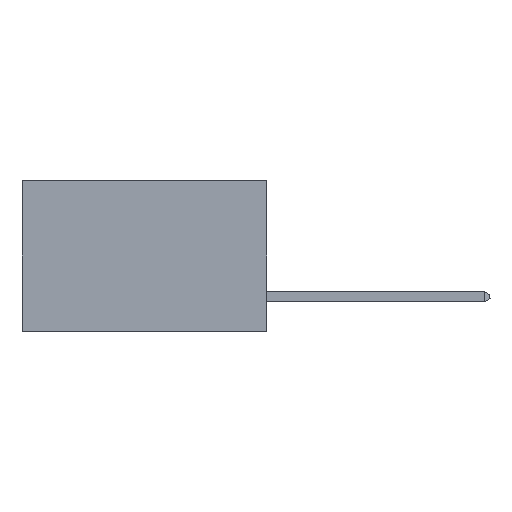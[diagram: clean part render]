
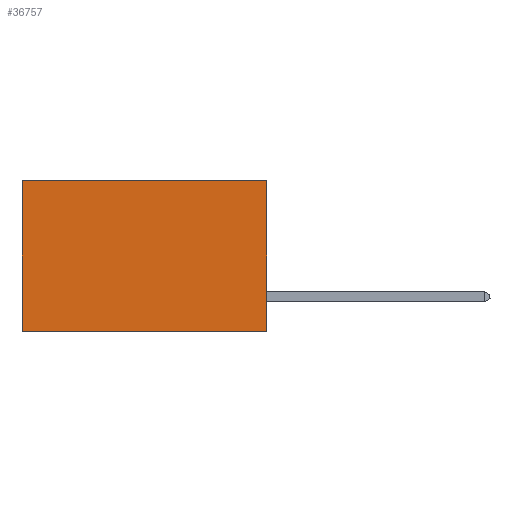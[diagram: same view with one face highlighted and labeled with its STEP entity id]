
A CAD part, left-side view. The second image highlights one B-rep face of the part: STEP entity #36757.
In plain terms, the highlighted planar face has unit normal (-1, 0, 0).
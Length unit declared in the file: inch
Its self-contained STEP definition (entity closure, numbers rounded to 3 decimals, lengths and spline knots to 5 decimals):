
#1251 = CARTESIAN_POINT ( 'NONE',  ( 0.2875, 0.6, 0. ) ) ;
#1369 = ORIENTED_EDGE ( 'NONE', *, *, #16127, .F. ) ;
#1934 = CARTESIAN_POINT ( 'NONE',  ( 0.2875, 0., -0.37 ) ) ;
#4135 = CARTESIAN_POINT ( 'NONE',  ( 0.2875, 0., -0.37 ) ) ;
#4582 = CARTESIAN_POINT ( 'NONE',  ( 0.2875, 0., 0. ) ) ;
#4763 = CARTESIAN_POINT ( 'NONE',  ( 0.2875, 0.6, 0. ) ) ;
#5867 = DIRECTION ( 'NONE',  ( 0., 1., 0. ) ) ;
#7836 = EDGE_CURVE ( 'NONE', #48244, #20547, #32743, .T. ) ;
#7892 = DIRECTION ( 'NONE',  ( 0., 0., -1. ) ) ;
#16127 = EDGE_CURVE ( 'NONE', #20547, #27169, #27175, .T. ) ;
#17280 = PLANE ( 'NONE',  #46109 ) ;
#17436 = DIRECTION ( 'NONE',  ( 1., 0., 0. ) ) ;
#17956 = ORIENTED_EDGE ( 'NONE', *, *, #19092, .T. ) ;
#18039 = VECTOR ( 'NONE', #7892, 39.37008 ) ;
#19092 = EDGE_CURVE ( 'NONE', #46174, #27169, #46648, .T. ) ;
#20547 = VERTEX_POINT ( 'NONE', #4135 ) ;
#22551 = CARTESIAN_POINT ( 'NONE',  ( 0.2875, 0., 0. ) ) ;
#25552 = DIRECTION ( 'NONE',  ( 0., 1., 0. ) ) ;
#27169 = VERTEX_POINT ( 'NONE', #30133 ) ;
#27175 = LINE ( 'NONE', #1934, #41879 ) ;
#27359 = FACE_OUTER_BOUND ( 'NONE', #40513, .T. ) ;
#30133 = CARTESIAN_POINT ( 'NONE',  ( 0.2875, 0.6, -0.37 ) ) ;
#30190 = LINE ( 'NONE', #22551, #39016 ) ;
#31877 = EDGE_CURVE ( 'NONE', #48244, #46174, #30190, .T. ) ;
#32434 = ORIENTED_EDGE ( 'NONE', *, *, #31877, .T. ) ;
#32743 = LINE ( 'NONE', #4582, #18039 ) ;
#35697 = CARTESIAN_POINT ( 'NONE',  ( 0.2875, 0., 0. ) ) ;
#36757 = ADVANCED_FACE ( 'NONE', ( #27359 ), #17280, .F. ) ;
#37189 = VECTOR ( 'NONE', #39236, 39.37008 ) ;
#39016 = VECTOR ( 'NONE', #25552, 39.37008 ) ;
#39236 = DIRECTION ( 'NONE',  ( 0., 0., -1. ) ) ;
#39994 = CARTESIAN_POINT ( 'NONE',  ( 0.2875, 0., 0. ) ) ;
#40513 = EDGE_LOOP ( 'NONE', ( #17956, #1369, #47783, #32434 ) ) ;
#41879 = VECTOR ( 'NONE', #5867, 39.37008 ) ;
#43769 = DIRECTION ( 'NONE',  ( 0., 0., -1. ) ) ;
#46109 = AXIS2_PLACEMENT_3D ( 'NONE', #39994, #17436, #43769 ) ;
#46174 = VERTEX_POINT ( 'NONE', #4763 ) ;
#46648 = LINE ( 'NONE', #1251, #37189 ) ;
#47783 = ORIENTED_EDGE ( 'NONE', *, *, #7836, .F. ) ;
#48244 = VERTEX_POINT ( 'NONE', #35697 ) ;
